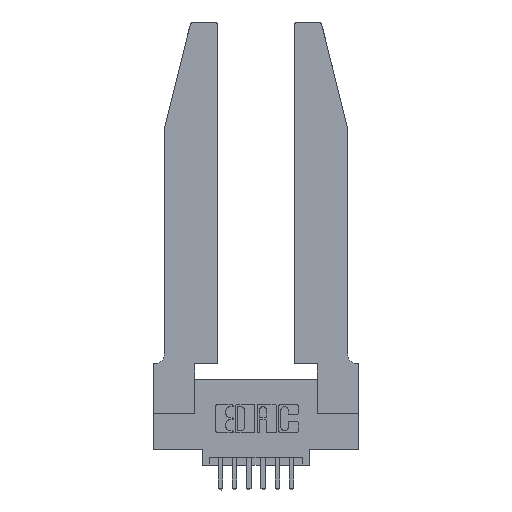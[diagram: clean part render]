
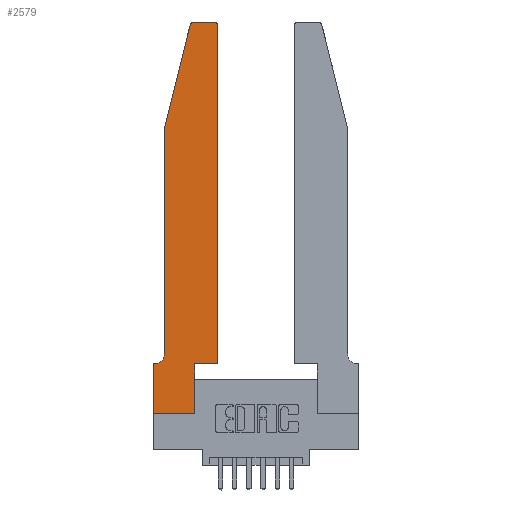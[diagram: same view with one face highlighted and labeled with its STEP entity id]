
A CAD part, top view. The second image highlights one B-rep face of the part: STEP entity #2579.
In plain terms, the highlighted planar face has unit normal (0, 0, 1).
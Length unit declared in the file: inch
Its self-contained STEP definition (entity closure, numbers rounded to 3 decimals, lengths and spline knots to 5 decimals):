
#582 = VECTOR ( 'NONE', #6304, 39.37008 ) ;
#629 = CARTESIAN_POINT ( 'NONE',  ( 0.0755, 0.35, 0.37 ) ) ;
#681 = EDGE_CURVE ( 'NONE', #10873, #6117, #8685, .T. ) ;
#702 = CARTESIAN_POINT ( 'NONE',  ( 0.0055, 0.35, 0.37 ) ) ;
#831 = ORIENTED_EDGE ( 'NONE', *, *, #681, .T. ) ;
#1038 = ORIENTED_EDGE ( 'NONE', *, *, #11661, .T. ) ;
#1093 = CARTESIAN_POINT ( 'NONE',  ( 0.2865, 0.35, 0.37 ) ) ;
#1125 = EDGE_CURVE ( 'NONE', #13796, #8285, #1135, .T. ) ;
#1135 = LINE ( 'NONE', #5267, #12384 ) ;
#1529 = ORIENTED_EDGE ( 'NONE', *, *, #1125, .T. ) ;
#1674 = DIRECTION ( 'NONE',  ( 0., 0., 1. ) ) ;
#1709 = ORIENTED_EDGE ( 'NONE', *, *, #9168, .T. ) ;
#1756 = DIRECTION ( 'NONE',  ( -1., 0., 0. ) ) ;
#1775 = CARTESIAN_POINT ( 'NONE',  ( 0.284, 2.75, 0.37 ) ) ;
#1777 = VECTOR ( 'NONE', #4967, 39.37008 ) ;
#1958 = CARTESIAN_POINT ( 'NONE',  ( 0.4505, 2.72, 0.37 ) ) ;
#2010 = CARTESIAN_POINT ( 'NONE',  ( 0.4505, 0.35, 0.37 ) ) ;
#2073 = CARTESIAN_POINT ( 'NONE',  ( 0.2605, 2.75, 0.37 ) ) ;
#2273 = DIRECTION ( 'NONE',  ( 0., 0., 1. ) ) ;
#2323 = CARTESIAN_POINT ( 'NONE',  ( 0., 0.35, 0.37 ) ) ;
#2530 = AXIS2_PLACEMENT_3D ( 'NONE', #2323, #2273, #10153 ) ;
#2579 = ADVANCED_FACE ( 'NONE', ( #8060 ), #7867, .T. ) ;
#2824 = VERTEX_POINT ( 'NONE', #11741 ) ;
#2890 = VERTEX_POINT ( 'NONE', #1958 ) ;
#2928 = LINE ( 'NONE', #2010, #14162 ) ;
#3058 = CIRCLE ( 'NONE', #12227, 0.03 ) ;
#3195 = VERTEX_POINT ( 'NONE', #702 ) ;
#3404 = CARTESIAN_POINT ( 'NONE',  ( 0.0055, 0.42, 0.37 ) ) ;
#3412 = ORIENTED_EDGE ( 'NONE', *, *, #5735, .T. ) ;
#3586 = EDGE_CURVE ( 'NONE', #12138, #3195, #12243, .T. ) ;
#3906 = CARTESIAN_POINT ( 'NONE',  ( 0.4505, 0.35, 0.37 ) ) ;
#4205 = DIRECTION ( 'NONE',  ( 0., 1., 0. ) ) ;
#4418 = EDGE_LOOP ( 'NONE', ( #12885, #13364, #6850, #8389, #5789, #1709, #831, #1038, #1529, #8608, #3412, #8234 ) ) ;
#4636 = EDGE_CURVE ( 'NONE', #8285, #2824, #2928, .T. ) ;
#4803 = VERTEX_POINT ( 'NONE', #6795 ) ;
#4967 = DIRECTION ( 'NONE',  ( -0.239, -0.971, 0. ) ) ;
#5267 = CARTESIAN_POINT ( 'NONE',  ( 0.2865, 0.35, 0.37 ) ) ;
#5325 = LINE ( 'NONE', #3906, #582 ) ;
#5435 = DIRECTION ( 'NONE',  ( 1., 0., 0. ) ) ;
#5693 = CARTESIAN_POINT ( 'NONE',  ( 0.0755, 0.42, 0.37 ) ) ;
#5735 = EDGE_CURVE ( 'NONE', #2824, #2890, #5325, .T. ) ;
#5789 = ORIENTED_EDGE ( 'NONE', *, *, #3586, .T. ) ;
#5933 = CARTESIAN_POINT ( 'NONE',  ( 0.25487, 2.72718, 0.37 ) ) ;
#6117 = VERTEX_POINT ( 'NONE', #10672 ) ;
#6304 = DIRECTION ( 'NONE',  ( 0., 1., 0. ) ) ;
#6408 = EDGE_CURVE ( 'NONE', #13604, #9221, #3058, .T. ) ;
#6486 = AXIS2_PLACEMENT_3D ( 'NONE', #3404, #11232, #10232 ) ;
#6534 = EDGE_CURVE ( 'NONE', #2890, #4803, #11296, .T. ) ;
#6795 = CARTESIAN_POINT ( 'NONE',  ( 0.4205, 2.75, 0.37 ) ) ;
#6850 = ORIENTED_EDGE ( 'NONE', *, *, #7264, .T. ) ;
#7115 = DIRECTION ( 'NONE',  ( 1., 0., 0. ) ) ;
#7264 = EDGE_CURVE ( 'NONE', #9221, #9359, #10204, .T. ) ;
#7278 = VECTOR ( 'NONE', #1756, 39.37008 ) ;
#7505 = VECTOR ( 'NONE', #12045, 39.37008 ) ;
#7867 = PLANE ( 'NONE',  #2530 ) ;
#8060 = FACE_OUTER_BOUND ( 'NONE', #4418, .T. ) ;
#8234 = ORIENTED_EDGE ( 'NONE', *, *, #6534, .T. ) ;
#8259 = LINE ( 'NONE', #13613, #14434 ) ;
#8285 = VERTEX_POINT ( 'NONE', #1093 ) ;
#8389 = ORIENTED_EDGE ( 'NONE', *, *, #10349, .T. ) ;
#8608 = ORIENTED_EDGE ( 'NONE', *, *, #4636, .T. ) ;
#8685 = LINE ( 'NONE', #11070, #14334 ) ;
#8785 = DIRECTION ( 'NONE',  ( 1., 0., 0. ) ) ;
#9168 = EDGE_CURVE ( 'NONE', #3195, #10873, #10922, .T. ) ;
#9221 = VERTEX_POINT ( 'NONE', #5933 ) ;
#9359 = VERTEX_POINT ( 'NONE', #9690 ) ;
#9690 = CARTESIAN_POINT ( 'NONE',  ( 0.0755, 2., 0.37 ) ) ;
#9883 = CARTESIAN_POINT ( 'NONE',  ( 0., 0.35, 0.37 ) ) ;
#9911 = LINE ( 'NONE', #2073, #7505 ) ;
#10153 = DIRECTION ( 'NONE',  ( 1., 0., 0. ) ) ;
#10168 = LINE ( 'NONE', #12156, #14405 ) ;
#10204 = LINE ( 'NONE', #11656, #1777 ) ;
#10232 = DIRECTION ( 'NONE',  ( -1., 0., 0. ) ) ;
#10349 = EDGE_CURVE ( 'NONE', #9359, #12138, #8259, .T. ) ;
#10672 = CARTESIAN_POINT ( 'NONE',  ( 0., 0., 0.37 ) ) ;
#10873 = VERTEX_POINT ( 'NONE', #9883 ) ;
#10922 = LINE ( 'NONE', #629, #7278 ) ;
#11070 = CARTESIAN_POINT ( 'NONE',  ( 0., 0., 0.37 ) ) ;
#11232 = DIRECTION ( 'NONE',  ( 0., 0., -1. ) ) ;
#11296 = CIRCLE ( 'NONE', #13004, 0.03 ) ;
#11656 = CARTESIAN_POINT ( 'NONE',  ( 0.0755, 2., 0.37 ) ) ;
#11661 = EDGE_CURVE ( 'NONE', #6117, #13796, #10168, .T. ) ;
#11741 = CARTESIAN_POINT ( 'NONE',  ( 0.4505, 0.35, 0.37 ) ) ;
#11792 = CARTESIAN_POINT ( 'NONE',  ( 0.4205, 2.72, 0.37 ) ) ;
#12045 = DIRECTION ( 'NONE',  ( -1., 0., 0. ) ) ;
#12138 = VERTEX_POINT ( 'NONE', #5693 ) ;
#12156 = CARTESIAN_POINT ( 'NONE',  ( 0., 0., 0.37 ) ) ;
#12227 = AXIS2_PLACEMENT_3D ( 'NONE', #12497, #13704, #7115 ) ;
#12230 = CARTESIAN_POINT ( 'NONE',  ( 0.2865, 0., 0.37 ) ) ;
#12243 = CIRCLE ( 'NONE', #6486, 0.07 ) ;
#12384 = VECTOR ( 'NONE', #4205, 39.37008 ) ;
#12497 = CARTESIAN_POINT ( 'NONE',  ( 0.284, 2.72, 0.37 ) ) ;
#12885 = ORIENTED_EDGE ( 'NONE', *, *, #13676, .T. ) ;
#13004 = AXIS2_PLACEMENT_3D ( 'NONE', #11792, #1674, #14062 ) ;
#13364 = ORIENTED_EDGE ( 'NONE', *, *, #6408, .T. ) ;
#13420 = DIRECTION ( 'NONE',  ( 0., -1., 0. ) ) ;
#13456 = DIRECTION ( 'NONE',  ( 0., -1., 0. ) ) ;
#13604 = VERTEX_POINT ( 'NONE', #1775 ) ;
#13613 = CARTESIAN_POINT ( 'NONE',  ( 0.0755, 2., 0.37 ) ) ;
#13676 = EDGE_CURVE ( 'NONE', #4803, #13604, #9911, .T. ) ;
#13704 = DIRECTION ( 'NONE',  ( 0., 0., 1. ) ) ;
#13796 = VERTEX_POINT ( 'NONE', #12230 ) ;
#14062 = DIRECTION ( 'NONE',  ( 1., 0., 0. ) ) ;
#14162 = VECTOR ( 'NONE', #8785, 39.37008 ) ;
#14334 = VECTOR ( 'NONE', #13420, 39.37008 ) ;
#14405 = VECTOR ( 'NONE', #5435, 39.37008 ) ;
#14434 = VECTOR ( 'NONE', #13456, 39.37008 ) ;
